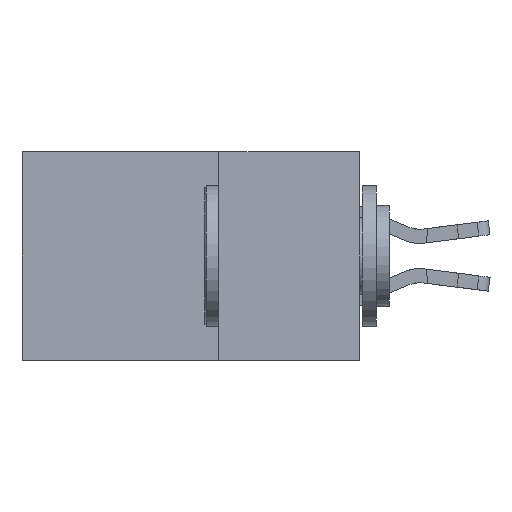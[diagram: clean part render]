
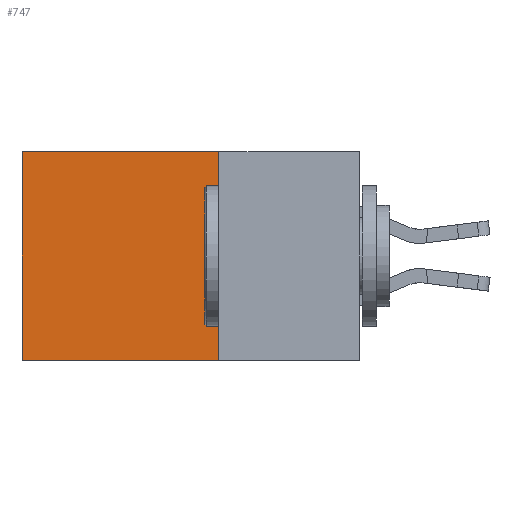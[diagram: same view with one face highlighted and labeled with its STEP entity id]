
A CAD part, left-side view. The second image highlights one B-rep face of the part: STEP entity #747.
In plain terms, the highlighted planar face has unit normal (-1, 0, 0).
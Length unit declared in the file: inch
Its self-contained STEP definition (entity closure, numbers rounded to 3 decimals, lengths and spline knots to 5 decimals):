
#444 = VERTEX_POINT ( 'NONE', #12678 ) ;
#706 = LINE ( 'NONE', #10839, #1194 ) ;
#747 = ADVANCED_FACE ( 'NONE', ( #11745 ), #18188, .F. ) ;
#1078 = ORIENTED_EDGE ( 'NONE', *, *, #6829, .T. ) ;
#1116 = CARTESIAN_POINT ( 'NONE',  ( 0.2875, 0.6, 0. ) ) ;
#1194 = VECTOR ( 'NONE', #3242, 39.37008 ) ;
#1645 = LINE ( 'NONE', #7008, #5802 ) ;
#2196 = ORIENTED_EDGE ( 'NONE', *, *, #5892, .T. ) ;
#3242 = DIRECTION ( 'NONE',  ( 0., 0., -1. ) ) ;
#4818 = LINE ( 'NONE', #5392, #16279 ) ;
#4966 = VERTEX_POINT ( 'NONE', #13510 ) ;
#5145 = CARTESIAN_POINT ( 'NONE',  ( 0.2875, 0.25, -0.37 ) ) ;
#5392 = CARTESIAN_POINT ( 'NONE',  ( 0.2875, 0.25, 0. ) ) ;
#5802 = VECTOR ( 'NONE', #10045, 39.37008 ) ;
#5892 = EDGE_CURVE ( 'NONE', #13908, #444, #1645, .T. ) ;
#6829 = EDGE_CURVE ( 'NONE', #18155, #13908, #4818, .T. ) ;
#6893 = DIRECTION ( 'NONE',  ( 0., 1., 0. ) ) ;
#7008 = CARTESIAN_POINT ( 'NONE',  ( 0.2875, 0.6, 0. ) ) ;
#7601 = ORIENTED_EDGE ( 'NONE', *, *, #19270, .F. ) ;
#8501 = EDGE_CURVE ( 'NONE', #4966, #444, #16978, .T. ) ;
#9266 = EDGE_LOOP ( 'NONE', ( #2196, #10870, #7601, #1078 ) ) ;
#10045 = DIRECTION ( 'NONE',  ( 0., 0., -1. ) ) ;
#10839 = CARTESIAN_POINT ( 'NONE',  ( 0.2875, 0.25, 0. ) ) ;
#10870 = ORIENTED_EDGE ( 'NONE', *, *, #8501, .F. ) ;
#11003 = CARTESIAN_POINT ( 'NONE',  ( 0.2875, 0.25, 0. ) ) ;
#11745 = FACE_OUTER_BOUND ( 'NONE', #9266, .T. ) ;
#12678 = CARTESIAN_POINT ( 'NONE',  ( 0.2875, 0.6, -0.37 ) ) ;
#13510 = CARTESIAN_POINT ( 'NONE',  ( 0.2875, 0.25, -0.37 ) ) ;
#13908 = VERTEX_POINT ( 'NONE', #1116 ) ;
#14106 = DIRECTION ( 'NONE',  ( 0., 1., 0. ) ) ;
#16041 = VECTOR ( 'NONE', #14106, 39.37008 ) ;
#16279 = VECTOR ( 'NONE', #6893, 39.37008 ) ;
#16978 = LINE ( 'NONE', #5145, #16041 ) ;
#17953 = AXIS2_PLACEMENT_3D ( 'NONE', #19623, #18552, #18580 ) ;
#18155 = VERTEX_POINT ( 'NONE', #11003 ) ;
#18188 = PLANE ( 'NONE',  #17953 ) ;
#18552 = DIRECTION ( 'NONE',  ( 1., 0., 0. ) ) ;
#18580 = DIRECTION ( 'NONE',  ( 0., 0., -1. ) ) ;
#19270 = EDGE_CURVE ( 'NONE', #18155, #4966, #706, .T. ) ;
#19623 = CARTESIAN_POINT ( 'NONE',  ( 0.2875, 0.25, 0. ) ) ;
